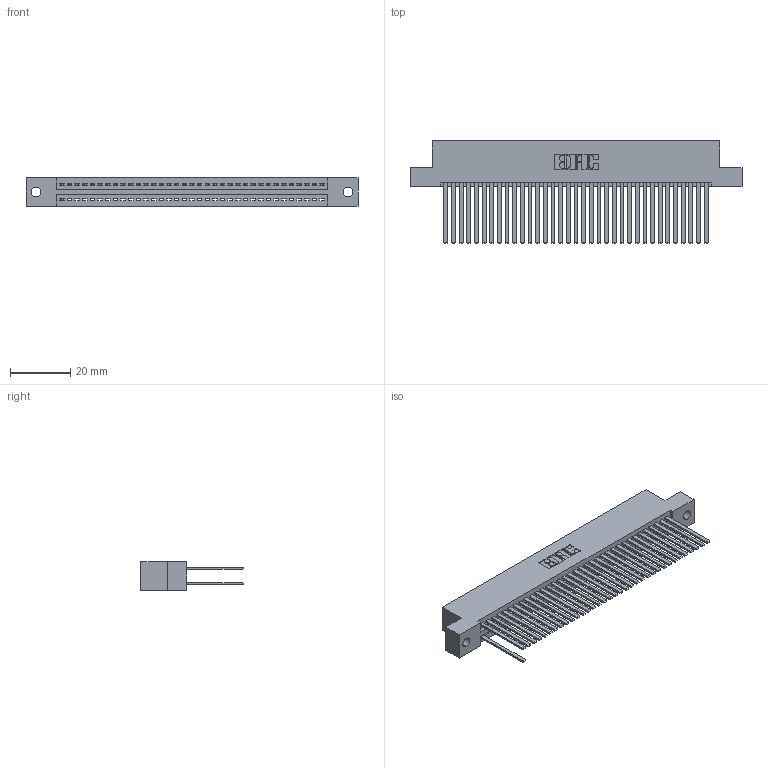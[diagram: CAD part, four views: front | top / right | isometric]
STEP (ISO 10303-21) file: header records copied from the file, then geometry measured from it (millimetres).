
FILE_DESCRIPTION (( 'STEP AP203' ), '1' );
FILE_NAME ('395-070-544-202.STEP', '2018-11-26T22:47:10', ( '' ), ( '' ), 'SwSTEP 2.0', 'SolidWorks 2016', '' );
FILE_SCHEMA (( 'CONFIG_CONTROL_DESIGN' ));
Length unit declared in the file: inch
Products named in the file (3): 345 Part_Flush Mounting Lugs - 0.128 Dia; 345-292-001_345-293-144; 395-070-544-202
Assembly tree (37 placements, depth 2):
  395-070-544-202
    345 Part_Flush Mounting Lugs - 0.128 Dia
    345-292-001_345-293-144  x36
Bounding box: 110.11 x 33.96 x 9.4 mm (x, y, z)
Volume: 10792.6 mm3; surface area: 15288.2 mm2
Topology: 37 solids, 37 shells, 1982 faces, 5975 edges, 3934 vertices
Faces by surface type: plane 1362, cylinder 620
Entity records: 27135 total; most frequent: CARTESIAN_POINT 4702, ORIENTED_EDGE 4670, DIRECTION 4115, EDGE_CURVE 2335, VECTOR 2067, LINE 2067, VERTEX_POINT 1554, AXIS2_PLACEMENT_3D 1024
